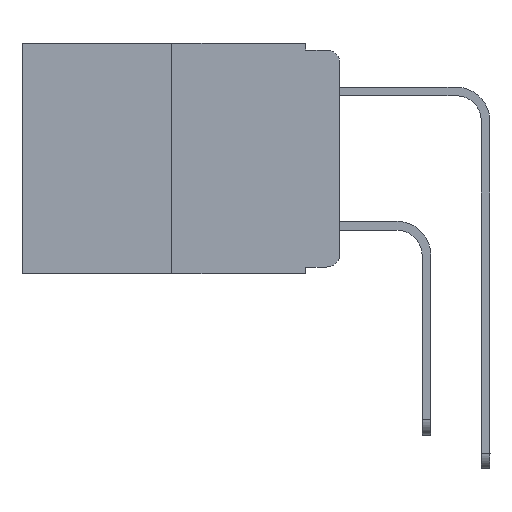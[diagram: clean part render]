
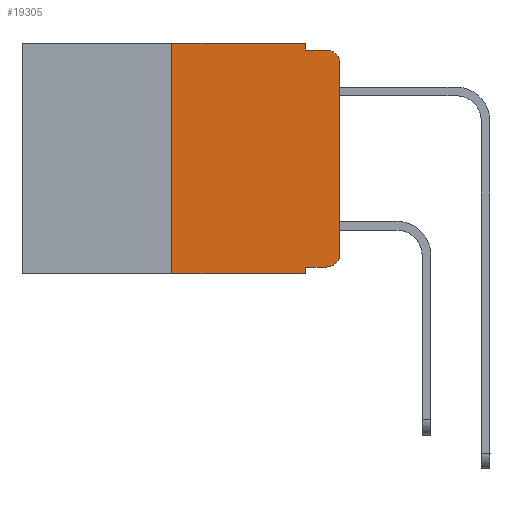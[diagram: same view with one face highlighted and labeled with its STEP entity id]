
A CAD part, left-side view. The second image highlights one B-rep face of the part: STEP entity #19305.
In plain terms, the highlighted planar face has unit normal (-1, 0, 0).
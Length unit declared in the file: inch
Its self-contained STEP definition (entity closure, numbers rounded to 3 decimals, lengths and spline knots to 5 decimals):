
#223 = EDGE_CURVE ( 'NONE', #2912, #22387, #5098, .T. ) ;
#291 = DIRECTION ( 'NONE',  ( 0., 0., -1. ) ) ;
#478 = AXIS2_PLACEMENT_3D ( 'NONE', #9113, #16364, #291 ) ;
#985 = EDGE_CURVE ( 'NONE', #15284, #12791, #20486, .T. ) ;
#1153 = ORIENTED_EDGE ( 'NONE', *, *, #8902, .T. ) ;
#1266 = CARTESIAN_POINT ( 'NONE',  ( 0., 0.051, 0. ) ) ;
#1736 = DIRECTION ( 'NONE',  ( -1., 0., 0. ) ) ;
#1988 = AXIS2_PLACEMENT_3D ( 'NONE', #6371, #7480, #18348 ) ;
#2004 = DIRECTION ( 'NONE',  ( 0., -1., 0. ) ) ;
#2099 = ORIENTED_EDGE ( 'NONE', *, *, #9924, .F. ) ;
#2267 = VERTEX_POINT ( 'NONE', #23006 ) ;
#2556 = VERTEX_POINT ( 'NONE', #7168 ) ;
#2564 = CIRCLE ( 'NONE', #10809, 0.02 ) ;
#2912 = VERTEX_POINT ( 'NONE', #22921 ) ;
#3329 = VECTOR ( 'NONE', #3500, 39.37008 ) ;
#3500 = DIRECTION ( 'NONE',  ( 0., 0., -1. ) ) ;
#3577 = ORIENTED_EDGE ( 'NONE', *, *, #13144, .T. ) ;
#3680 = CARTESIAN_POINT ( 'NONE',  ( 0., 0.051, -0.343 ) ) ;
#3948 = VERTEX_POINT ( 'NONE', #16080 ) ;
#3952 = FACE_OUTER_BOUND ( 'NONE', #16844, .T. ) ;
#4505 = VECTOR ( 'NONE', #2004, 39.37008 ) ;
#4589 = CIRCLE ( 'NONE', #1988, 0.02 ) ;
#5098 = LINE ( 'NONE', #6986, #22988 ) ;
#5682 = EDGE_CURVE ( 'NONE', #15250, #12791, #21213, .T. ) ;
#5755 = EDGE_CURVE ( 'NONE', #15284, #2556, #15948, .T. ) ;
#5826 = PLANE ( 'NONE',  #478 ) ;
#6296 = DIRECTION ( 'NONE',  ( 0., 0., 1. ) ) ;
#6309 = VERTEX_POINT ( 'NONE', #22538 ) ;
#6336 = CARTESIAN_POINT ( 'NONE',  ( 0., 0.051, 0. ) ) ;
#6371 = CARTESIAN_POINT ( 'NONE',  ( 0., 0.02, -0.313 ) ) ;
#6906 = LINE ( 'NONE', #1266, #3329 ) ;
#6986 = CARTESIAN_POINT ( 'NONE',  ( 0., 0.051, -0.01 ) ) ;
#7168 = CARTESIAN_POINT ( 'NONE',  ( 0., 0.02, -0.333 ) ) ;
#7178 = DIRECTION ( 'NONE',  ( 0., -1., 0. ) ) ;
#7480 = DIRECTION ( 'NONE',  ( -1., 0., 0. ) ) ;
#8017 = VECTOR ( 'NONE', #9129, 39.37008 ) ;
#8061 = CARTESIAN_POINT ( 'NONE',  ( 0., 0.25, 0. ) ) ;
#8331 = DIRECTION ( 'NONE',  ( 0., 0., -1. ) ) ;
#8733 = VECTOR ( 'NONE', #13668, 39.37008 ) ;
#8902 = EDGE_CURVE ( 'NONE', #2267, #6309, #12266, .T. ) ;
#8910 = ORIENTED_EDGE ( 'NONE', *, *, #13168, .F. ) ;
#9113 = CARTESIAN_POINT ( 'NONE',  ( 0., 0.473, 0. ) ) ;
#9116 = ORIENTED_EDGE ( 'NONE', *, *, #9881, .F. ) ;
#9129 = DIRECTION ( 'NONE',  ( 0., -1., 0. ) ) ;
#9352 = CARTESIAN_POINT ( 'NONE',  ( 0., 0.473, 0. ) ) ;
#9694 = CARTESIAN_POINT ( 'NONE',  ( 0., 0.02, -0.01 ) ) ;
#9881 = EDGE_CURVE ( 'NONE', #20327, #3948, #17909, .T. ) ;
#9924 = EDGE_CURVE ( 'NONE', #15250, #20327, #13322, .T. ) ;
#10185 = CARTESIAN_POINT ( 'NONE',  ( 0., 0.02, -0.03 ) ) ;
#10694 = CARTESIAN_POINT ( 'NONE',  ( 0., 0.473, -0.343 ) ) ;
#10809 = AXIS2_PLACEMENT_3D ( 'NONE', #10185, #1736, #14162 ) ;
#11480 = ORIENTED_EDGE ( 'NONE', *, *, #985, .F. ) ;
#11759 = CARTESIAN_POINT ( 'NONE',  ( 0., 0.051, -0.333 ) ) ;
#11762 = ORIENTED_EDGE ( 'NONE', *, *, #223, .F. ) ;
#12248 = VECTOR ( 'NONE', #8331, 39.37008 ) ;
#12266 = LINE ( 'NONE', #15405, #8733 ) ;
#12791 = VERTEX_POINT ( 'NONE', #3680 ) ;
#13144 = EDGE_CURVE ( 'NONE', #6309, #22387, #2564, .T. ) ;
#13168 = EDGE_CURVE ( 'NONE', #3948, #2912, #6906, .T. ) ;
#13322 = LINE ( 'NONE', #8061, #22198 ) ;
#13668 = DIRECTION ( 'NONE',  ( 0., 0., 1. ) ) ;
#14162 = DIRECTION ( 'NONE',  ( 0., 0., -1. ) ) ;
#14611 = VECTOR ( 'NONE', #7178, 39.37008 ) ;
#15250 = VERTEX_POINT ( 'NONE', #15714 ) ;
#15284 = VERTEX_POINT ( 'NONE', #11759 ) ;
#15405 = CARTESIAN_POINT ( 'NONE',  ( 0., 0., 0. ) ) ;
#15518 = ORIENTED_EDGE ( 'NONE', *, *, #5682, .T. ) ;
#15714 = CARTESIAN_POINT ( 'NONE',  ( 0., 0.25, -0.343 ) ) ;
#15948 = LINE ( 'NONE', #16301, #14611 ) ;
#16080 = CARTESIAN_POINT ( 'NONE',  ( 0., 0.051, 0. ) ) ;
#16301 = CARTESIAN_POINT ( 'NONE',  ( 0., 0.051, -0.333 ) ) ;
#16309 = CARTESIAN_POINT ( 'NONE',  ( 0., 0.25, 0. ) ) ;
#16364 = DIRECTION ( 'NONE',  ( 1., 0., 0. ) ) ;
#16844 = EDGE_LOOP ( 'NONE', ( #1153, #3577, #11762, #8910, #9116, #2099, #15518, #11480, #18896, #19828 ) ) ;
#17725 = EDGE_CURVE ( 'NONE', #2556, #2267, #4589, .T. ) ;
#17909 = LINE ( 'NONE', #9352, #8017 ) ;
#18348 = DIRECTION ( 'NONE',  ( 0., 0., -1. ) ) ;
#18896 = ORIENTED_EDGE ( 'NONE', *, *, #5755, .T. ) ;
#19305 = ADVANCED_FACE ( 'NONE', ( #3952 ), #5826, .F. ) ;
#19479 = DIRECTION ( 'NONE',  ( 0., -1., 0. ) ) ;
#19828 = ORIENTED_EDGE ( 'NONE', *, *, #17725, .T. ) ;
#20327 = VERTEX_POINT ( 'NONE', #16309 ) ;
#20486 = LINE ( 'NONE', #6336, #12248 ) ;
#21213 = LINE ( 'NONE', #10694, #4505 ) ;
#22198 = VECTOR ( 'NONE', #6296, 39.37008 ) ;
#22387 = VERTEX_POINT ( 'NONE', #9694 ) ;
#22538 = CARTESIAN_POINT ( 'NONE',  ( 0., 0., -0.03 ) ) ;
#22921 = CARTESIAN_POINT ( 'NONE',  ( 0., 0.051, -0.01 ) ) ;
#22988 = VECTOR ( 'NONE', #19479, 39.37008 ) ;
#23006 = CARTESIAN_POINT ( 'NONE',  ( 0., 0., -0.313 ) ) ;
